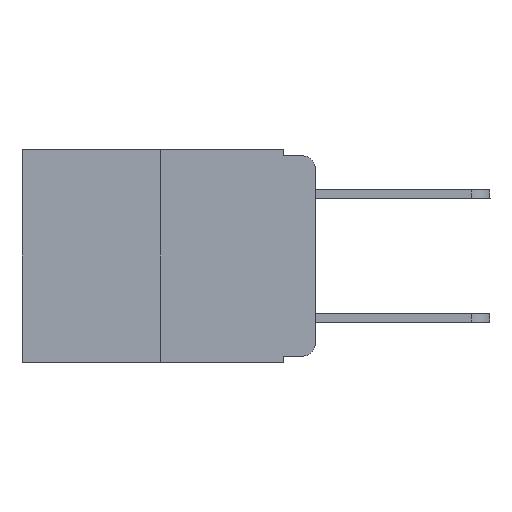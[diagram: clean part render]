
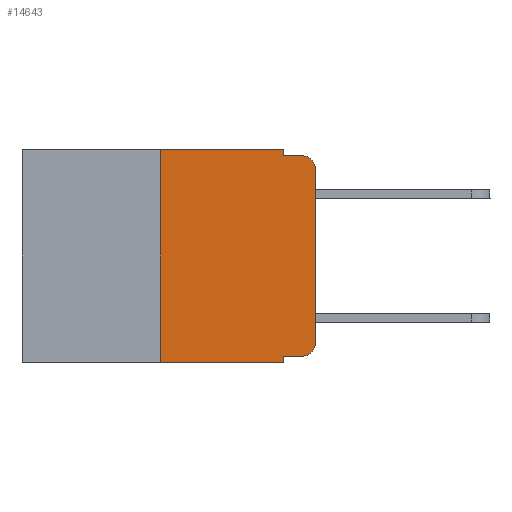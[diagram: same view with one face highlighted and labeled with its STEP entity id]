
A CAD part, left-side view. The second image highlights one B-rep face of the part: STEP entity #14643.
In plain terms, the highlighted planar face has unit normal (-1, 0, 0).
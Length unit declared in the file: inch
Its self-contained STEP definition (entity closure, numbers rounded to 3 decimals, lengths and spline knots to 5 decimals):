
#430 = ORIENTED_EDGE ( 'NONE', *, *, #17480, .T. ) ;
#440 = AXIS2_PLACEMENT_3D ( 'NONE', #16208, #14371, #8808 ) ;
#698 = AXIS2_PLACEMENT_3D ( 'NONE', #6574, #6865, #18207 ) ;
#894 = VERTEX_POINT ( 'NONE', #7450 ) ;
#960 = LINE ( 'NONE', #2671, #3110 ) ;
#1064 = CARTESIAN_POINT ( 'NONE',  ( 0., 0.02, -0.313 ) ) ;
#1286 = EDGE_CURVE ( 'NONE', #10369, #18215, #11471, .T. ) ;
#1353 = CARTESIAN_POINT ( 'NONE',  ( 0., 0.051, -0.333 ) ) ;
#1541 = ORIENTED_EDGE ( 'NONE', *, *, #10456, .T. ) ;
#1685 = CARTESIAN_POINT ( 'NONE',  ( 0., 0.25, 0. ) ) ;
#1997 = VERTEX_POINT ( 'NONE', #6151 ) ;
#2108 = EDGE_CURVE ( 'NONE', #18215, #8807, #960, .T. ) ;
#2614 = DIRECTION ( 'NONE',  ( 0., -1., 0. ) ) ;
#2671 = CARTESIAN_POINT ( 'NONE',  ( 0., 0.473, 0. ) ) ;
#2710 = LINE ( 'NONE', #5380, #3312 ) ;
#3110 = VECTOR ( 'NONE', #6976, 39.37008 ) ;
#3199 = CARTESIAN_POINT ( 'NONE',  ( 0., 0.051, -0.01 ) ) ;
#3312 = VECTOR ( 'NONE', #2614, 39.37008 ) ;
#3870 = PLANE ( 'NONE',  #698 ) ;
#4738 = DIRECTION ( 'NONE',  ( 0., 0., -1. ) ) ;
#4762 = LINE ( 'NONE', #15905, #6433 ) ;
#5288 = AXIS2_PLACEMENT_3D ( 'NONE', #1064, #11024, #16896 ) ;
#5380 = CARTESIAN_POINT ( 'NONE',  ( 0., 0.473, -0.343 ) ) ;
#5490 = CARTESIAN_POINT ( 'NONE',  ( 0., 0.051, 0. ) ) ;
#5577 = VECTOR ( 'NONE', #17885, 39.37008 ) ;
#5602 = ORIENTED_EDGE ( 'NONE', *, *, #16864, .F. ) ;
#5903 = CARTESIAN_POINT ( 'NONE',  ( 0., 0.051, 0. ) ) ;
#5968 = LINE ( 'NONE', #11841, #5577 ) ;
#6151 = CARTESIAN_POINT ( 'NONE',  ( 0., 0.051, -0.333 ) ) ;
#6343 = CARTESIAN_POINT ( 'NONE',  ( 0., 0.051, 0. ) ) ;
#6433 = VECTOR ( 'NONE', #8799, 39.37008 ) ;
#6450 = EDGE_LOOP ( 'NONE', ( #12663, #430, #15874, #6719, #18013, #18788, #1541, #5602, #12149, #14239 ) ) ;
#6574 = CARTESIAN_POINT ( 'NONE',  ( 0., 0.473, 0. ) ) ;
#6719 = ORIENTED_EDGE ( 'NONE', *, *, #9722, .F. ) ;
#6865 = DIRECTION ( 'NONE',  ( 1., 0., 0. ) ) ;
#6871 = CARTESIAN_POINT ( 'NONE',  ( 0., 0.02, -0.01 ) ) ;
#6976 = DIRECTION ( 'NONE',  ( 0., -1., 0. ) ) ;
#7075 = VECTOR ( 'NONE', #7193, 39.37008 ) ;
#7193 = DIRECTION ( 'NONE',  ( 0., -1., 0. ) ) ;
#7256 = VERTEX_POINT ( 'NONE', #7995 ) ;
#7450 = CARTESIAN_POINT ( 'NONE',  ( 0., 0.051, -0.343 ) ) ;
#7995 = CARTESIAN_POINT ( 'NONE',  ( 0., 0., -0.313 ) ) ;
#8329 = VECTOR ( 'NONE', #10949, 39.37008 ) ;
#8581 = VECTOR ( 'NONE', #13376, 39.37008 ) ;
#8799 = DIRECTION ( 'NONE',  ( 0., -1., 0. ) ) ;
#8807 = VERTEX_POINT ( 'NONE', #5490 ) ;
#8808 = DIRECTION ( 'NONE',  ( 0., 0., -1. ) ) ;
#9722 = EDGE_CURVE ( 'NONE', #8807, #16602, #13298, .T. ) ;
#10369 = VERTEX_POINT ( 'NONE', #12784 ) ;
#10456 = EDGE_CURVE ( 'NONE', #10369, #894, #2710, .T. ) ;
#10949 = DIRECTION ( 'NONE',  ( 0., 0., -1. ) ) ;
#11024 = DIRECTION ( 'NONE',  ( -1., 0., 0. ) ) ;
#11471 = LINE ( 'NONE', #1685, #8581 ) ;
#11734 = VERTEX_POINT ( 'NONE', #15759 ) ;
#11841 = CARTESIAN_POINT ( 'NONE',  ( 0., 0., 0. ) ) ;
#11875 = CARTESIAN_POINT ( 'NONE',  ( 0., 0., -0.03 ) ) ;
#12149 = ORIENTED_EDGE ( 'NONE', *, *, #14044, .T. ) ;
#12663 = ORIENTED_EDGE ( 'NONE', *, *, #16656, .T. ) ;
#12784 = CARTESIAN_POINT ( 'NONE',  ( 0., 0.25, -0.343 ) ) ;
#13022 = EDGE_CURVE ( 'NONE', #16602, #17809, #4762, .T. ) ;
#13249 = VERTEX_POINT ( 'NONE', #11875 ) ;
#13298 = LINE ( 'NONE', #5903, #13542 ) ;
#13376 = DIRECTION ( 'NONE',  ( 0., 0., 1. ) ) ;
#13542 = VECTOR ( 'NONE', #4738, 39.37008 ) ;
#14044 = EDGE_CURVE ( 'NONE', #1997, #11734, #14488, .T. ) ;
#14239 = ORIENTED_EDGE ( 'NONE', *, *, #17432, .T. ) ;
#14371 = DIRECTION ( 'NONE',  ( -1., 0., 0. ) ) ;
#14488 = LINE ( 'NONE', #1353, #7075 ) ;
#14643 = ADVANCED_FACE ( 'NONE', ( #17056 ), #3870, .F. ) ;
#15759 = CARTESIAN_POINT ( 'NONE',  ( 0., 0.02, -0.333 ) ) ;
#15874 = ORIENTED_EDGE ( 'NONE', *, *, #13022, .F. ) ;
#15905 = CARTESIAN_POINT ( 'NONE',  ( 0., 0.051, -0.01 ) ) ;
#16208 = CARTESIAN_POINT ( 'NONE',  ( 0., 0.02, -0.03 ) ) ;
#16602 = VERTEX_POINT ( 'NONE', #3199 ) ;
#16636 = LINE ( 'NONE', #6343, #8329 ) ;
#16656 = EDGE_CURVE ( 'NONE', #7256, #13249, #5968, .T. ) ;
#16662 = CIRCLE ( 'NONE', #440, 0.02 ) ;
#16864 = EDGE_CURVE ( 'NONE', #1997, #894, #16636, .T. ) ;
#16896 = DIRECTION ( 'NONE',  ( 0., 0., -1. ) ) ;
#17015 = CARTESIAN_POINT ( 'NONE',  ( 0., 0.25, 0. ) ) ;
#17056 = FACE_OUTER_BOUND ( 'NONE', #6450, .T. ) ;
#17272 = CIRCLE ( 'NONE', #5288, 0.02 ) ;
#17432 = EDGE_CURVE ( 'NONE', #11734, #7256, #17272, .T. ) ;
#17480 = EDGE_CURVE ( 'NONE', #13249, #17809, #16662, .T. ) ;
#17809 = VERTEX_POINT ( 'NONE', #6871 ) ;
#17885 = DIRECTION ( 'NONE',  ( 0., 0., 1. ) ) ;
#18013 = ORIENTED_EDGE ( 'NONE', *, *, #2108, .F. ) ;
#18207 = DIRECTION ( 'NONE',  ( 0., 0., -1. ) ) ;
#18215 = VERTEX_POINT ( 'NONE', #17015 ) ;
#18788 = ORIENTED_EDGE ( 'NONE', *, *, #1286, .F. ) ;
